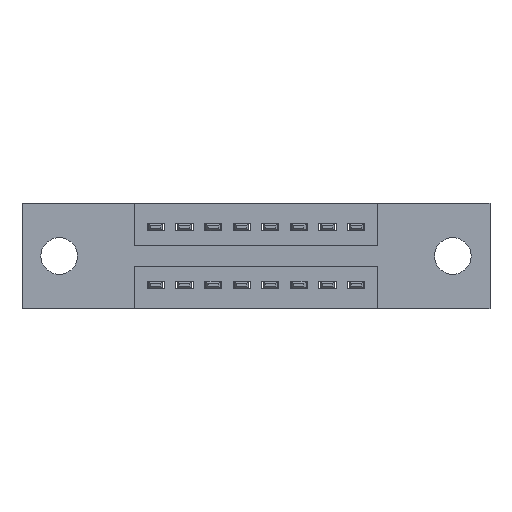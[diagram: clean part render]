
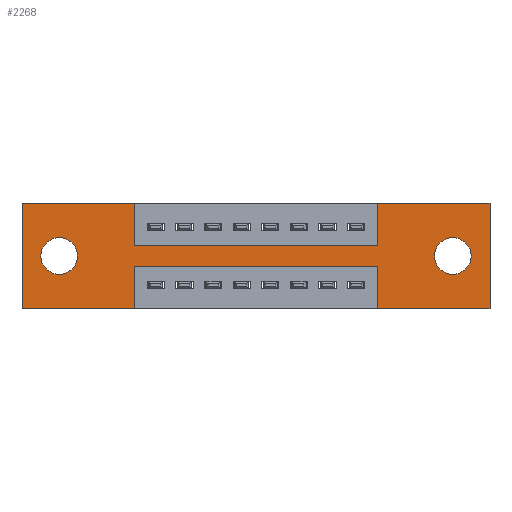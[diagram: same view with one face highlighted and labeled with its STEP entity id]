
A CAD part, front view. The second image highlights one B-rep face of the part: STEP entity #2268.
In plain terms, the highlighted planar face has unit normal (0, -1, 0).
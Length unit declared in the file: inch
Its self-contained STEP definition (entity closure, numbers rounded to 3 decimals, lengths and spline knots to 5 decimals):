
#105 = CARTESIAN_POINT ( 'NONE',  ( 0.3925, 0., -0.15 ) ) ;
#108 = CARTESIAN_POINT ( 'NONE',  ( 0.13, 0., -0.121 ) ) ;
#109 = FACE_BOUND ( 'NONE', #9488, .T. ) ;
#119 = DIRECTION ( 'NONE',  ( 0., -1., 0. ) ) ;
#205 = VERTEX_POINT ( 'NONE', #1158 ) ;
#261 = CARTESIAN_POINT ( 'NONE',  ( 0.13, 0., -0.249 ) ) ;
#336 = ORIENTED_EDGE ( 'NONE', *, *, #9798, .T. ) ;
#409 = CARTESIAN_POINT ( 'NONE',  ( 1.505, 0., -0.249 ) ) ;
#481 = DIRECTION ( 'NONE',  ( 1., 0., 0. ) ) ;
#488 = ORIENTED_EDGE ( 'NONE', *, *, #3546, .T. ) ;
#514 = LINE ( 'NONE', #9756, #5161 ) ;
#735 = CARTESIAN_POINT ( 'NONE',  ( 1.2425, 0., -0.37 ) ) ;
#747 = DIRECTION ( 'NONE',  ( 0., 0., -1. ) ) ;
#782 = DIRECTION ( 'NONE',  ( 0., 1., 0. ) ) ;
#883 = ORIENTED_EDGE ( 'NONE', *, *, #3444, .T. ) ;
#1049 = CARTESIAN_POINT ( 'NONE',  ( 0.3925, 0., 0. ) ) ;
#1069 = ORIENTED_EDGE ( 'NONE', *, *, #6286, .T. ) ;
#1088 = AXIS2_PLACEMENT_3D ( 'NONE', #8961, #8933, #3361 ) ;
#1124 = LINE ( 'NONE', #8609, #5435 ) ;
#1139 = EDGE_CURVE ( 'NONE', #6554, #6584, #8208, .T. ) ;
#1158 = CARTESIAN_POINT ( 'NONE',  ( 1.635, 0., -0.37 ) ) ;
#1349 = CARTESIAN_POINT ( 'NONE',  ( 1.505, 0., -0.185 ) ) ;
#1469 = EDGE_CURVE ( 'NONE', #1929, #6581, #5214, .T. ) ;
#1492 = VECTOR ( 'NONE', #3871, 39.37008 ) ;
#1554 = CARTESIAN_POINT ( 'NONE',  ( 1.2425, 0., -0.37 ) ) ;
#1603 = CIRCLE ( 'NONE', #6537, 0.064 ) ;
#1689 = CIRCLE ( 'NONE', #8355, 0.064 ) ;
#1772 = DIRECTION ( 'NONE',  ( 0., 0., 1. ) ) ;
#1795 = ORIENTED_EDGE ( 'NONE', *, *, #5296, .F. ) ;
#1887 = EDGE_CURVE ( 'NONE', #6584, #9141, #3772, .T. ) ;
#1929 = VERTEX_POINT ( 'NONE', #10676 ) ;
#1947 = VERTEX_POINT ( 'NONE', #261 ) ;
#2009 = EDGE_CURVE ( 'NONE', #8185, #10488, #4673, .T. ) ;
#2061 = ORIENTED_EDGE ( 'NONE', *, *, #1469, .F. ) ;
#2156 = ORIENTED_EDGE ( 'NONE', *, *, #2302, .F. ) ;
#2198 = ORIENTED_EDGE ( 'NONE', *, *, #3148, .F. ) ;
#2257 = DIRECTION ( 'NONE',  ( 0., 0., -1. ) ) ;
#2268 = ADVANCED_FACE ( 'NONE', ( #109, #2272, #6716 ), #5125, .T. ) ;
#2272 = FACE_BOUND ( 'NONE', #4322, .T. ) ;
#2302 = EDGE_CURVE ( 'NONE', #8116, #1929, #10304, .T. ) ;
#2501 = ORIENTED_EDGE ( 'NONE', *, *, #7516, .F. ) ;
#2599 = DIRECTION ( 'NONE',  ( 0., 0., -1. ) ) ;
#2653 = CARTESIAN_POINT ( 'NONE',  ( 1.2425, 0., 0. ) ) ;
#2776 = ORIENTED_EDGE ( 'NONE', *, *, #2009, .F. ) ;
#2954 = CARTESIAN_POINT ( 'NONE',  ( 0.3925, 0., 0. ) ) ;
#2968 = DIRECTION ( 'NONE',  ( 0., 0., 1. ) ) ;
#3147 = ORIENTED_EDGE ( 'NONE', *, *, #5895, .F. ) ;
#3148 = EDGE_CURVE ( 'NONE', #205, #8116, #6696, .T. ) ;
#3301 = ORIENTED_EDGE ( 'NONE', *, *, #1887, .F. ) ;
#3313 = ORIENTED_EDGE ( 'NONE', *, *, #1139, .F. ) ;
#3316 = CARTESIAN_POINT ( 'NONE',  ( 0.3925, 0., -0.37 ) ) ;
#3361 = DIRECTION ( 'NONE',  ( 0., 0., -1. ) ) ;
#3444 = EDGE_CURVE ( 'NONE', #8309, #1947, #8162, .T. ) ;
#3546 = EDGE_CURVE ( 'NONE', #7913, #3805, #6931, .T. ) ;
#3663 = VECTOR ( 'NONE', #747, 39.37008 ) ;
#3709 = ORIENTED_EDGE ( 'NONE', *, *, #8189, .F. ) ;
#3745 = VECTOR ( 'NONE', #1772, 39.37008 ) ;
#3772 = LINE ( 'NONE', #105, #5699 ) ;
#3793 = CARTESIAN_POINT ( 'NONE',  ( 0.3925, 0., -0.37 ) ) ;
#3805 = VERTEX_POINT ( 'NONE', #5075 ) ;
#3837 = CARTESIAN_POINT ( 'NONE',  ( 0.3925, 0., -0.15 ) ) ;
#3871 = DIRECTION ( 'NONE',  ( 0., 0., -1. ) ) ;
#3965 = VECTOR ( 'NONE', #4348, 39.37008 ) ;
#3995 = LINE ( 'NONE', #9830, #3745 ) ;
#4322 = EDGE_LOOP ( 'NONE', ( #883, #1069 ) ) ;
#4336 = ORIENTED_EDGE ( 'NONE', *, *, #6980, .F. ) ;
#4348 = DIRECTION ( 'NONE',  ( 1., 0., 0. ) ) ;
#4493 = VERTEX_POINT ( 'NONE', #8219 ) ;
#4520 = VECTOR ( 'NONE', #9313, 39.37008 ) ;
#4601 = VERTEX_POINT ( 'NONE', #7735 ) ;
#4673 = LINE ( 'NONE', #10606, #7091 ) ;
#4865 = LINE ( 'NONE', #8209, #7015 ) ;
#5075 = CARTESIAN_POINT ( 'NONE',  ( 1.505, 0., -0.121 ) ) ;
#5125 = PLANE ( 'NONE',  #9767 ) ;
#5161 = VECTOR ( 'NONE', #2599, 39.37008 ) ;
#5214 = LINE ( 'NONE', #9081, #5464 ) ;
#5296 = EDGE_CURVE ( 'NONE', #6581, #7438, #7876, .T. ) ;
#5390 = ORIENTED_EDGE ( 'NONE', *, *, #8733, .F. ) ;
#5435 = VECTOR ( 'NONE', #2968, 39.37008 ) ;
#5464 = VECTOR ( 'NONE', #9623, 39.37008 ) ;
#5699 = VECTOR ( 'NONE', #481, 39.37008 ) ;
#5827 = CARTESIAN_POINT ( 'NONE',  ( 1.635, 0., 0. ) ) ;
#5895 = EDGE_CURVE ( 'NONE', #9141, #8185, #1124, .T. ) ;
#5936 = CARTESIAN_POINT ( 'NONE',  ( 0.13, 0., -0.185 ) ) ;
#6159 = LINE ( 'NONE', #10601, #3965 ) ;
#6286 = EDGE_CURVE ( 'NONE', #1947, #8309, #1689, .T. ) ;
#6455 = VECTOR ( 'NONE', #6826, 39.37008 ) ;
#6537 = AXIS2_PLACEMENT_3D ( 'NONE', #1349, #7232, #2257 ) ;
#6554 = VERTEX_POINT ( 'NONE', #2954 ) ;
#6581 = VERTEX_POINT ( 'NONE', #8629 ) ;
#6584 = VERTEX_POINT ( 'NONE', #3837 ) ;
#6626 = DIRECTION ( 'NONE',  ( -1., 0., 0. ) ) ;
#6696 = LINE ( 'NONE', #9299, #4520 ) ;
#6716 = FACE_OUTER_BOUND ( 'NONE', #7766, .T. ) ;
#6740 = DIRECTION ( 'NONE',  ( 0., 0., 1. ) ) ;
#6784 = DIRECTION ( 'NONE',  ( 0., 0., -1. ) ) ;
#6826 = DIRECTION ( 'NONE',  ( 0., 0., 1. ) ) ;
#6931 = CIRCLE ( 'NONE', #1088, 0.064 ) ;
#6966 = AXIS2_PLACEMENT_3D ( 'NONE', #9503, #10080, #9565 ) ;
#6980 = EDGE_CURVE ( 'NONE', #4493, #4601, #3995, .T. ) ;
#7015 = VECTOR ( 'NONE', #6626, 39.37008 ) ;
#7091 = VECTOR ( 'NONE', #10526, 39.37008 ) ;
#7232 = DIRECTION ( 'NONE',  ( 0., 1., 0. ) ) ;
#7438 = VERTEX_POINT ( 'NONE', #3316 ) ;
#7516 = EDGE_CURVE ( 'NONE', #10488, #205, #514, .T. ) ;
#7735 = CARTESIAN_POINT ( 'NONE',  ( 0., 0., 0. ) ) ;
#7766 = EDGE_LOOP ( 'NONE', ( #1795, #2061, #2156, #2198, #2501, #2776, #3147, #3301, #3313, #3709, #4336, #5390 ) ) ;
#7876 = LINE ( 'NONE', #3793, #1492 ) ;
#7894 = CARTESIAN_POINT ( 'NONE',  ( 0., 0., -0.37 ) ) ;
#7913 = VERTEX_POINT ( 'NONE', #409 ) ;
#8116 = VERTEX_POINT ( 'NONE', #735 ) ;
#8162 = CIRCLE ( 'NONE', #6966, 0.064 ) ;
#8185 = VERTEX_POINT ( 'NONE', #2653 ) ;
#8189 = EDGE_CURVE ( 'NONE', #4601, #6554, #6159, .T. ) ;
#8208 = LINE ( 'NONE', #1049, #3663 ) ;
#8209 = CARTESIAN_POINT ( 'NONE',  ( 0., 0., -0.37 ) ) ;
#8219 = CARTESIAN_POINT ( 'NONE',  ( 0., 0., -0.37 ) ) ;
#8309 = VERTEX_POINT ( 'NONE', #108 ) ;
#8355 = AXIS2_PLACEMENT_3D ( 'NONE', #5936, #782, #6740 ) ;
#8609 = CARTESIAN_POINT ( 'NONE',  ( 1.2425, 0., 0. ) ) ;
#8629 = CARTESIAN_POINT ( 'NONE',  ( 0.3925, 0., -0.22 ) ) ;
#8716 = CARTESIAN_POINT ( 'NONE',  ( 1.2425, 0., -0.15 ) ) ;
#8733 = EDGE_CURVE ( 'NONE', #7438, #4493, #4865, .T. ) ;
#8933 = DIRECTION ( 'NONE',  ( 0., 1., 0. ) ) ;
#8961 = CARTESIAN_POINT ( 'NONE',  ( 1.505, 0., -0.185 ) ) ;
#9081 = CARTESIAN_POINT ( 'NONE',  ( 0.3925, 0., -0.22 ) ) ;
#9141 = VERTEX_POINT ( 'NONE', #8716 ) ;
#9299 = CARTESIAN_POINT ( 'NONE',  ( 0., 0., -0.37 ) ) ;
#9313 = DIRECTION ( 'NONE',  ( -1., 0., 0. ) ) ;
#9488 = EDGE_LOOP ( 'NONE', ( #336, #488 ) ) ;
#9503 = CARTESIAN_POINT ( 'NONE',  ( 0.13, 0., -0.185 ) ) ;
#9565 = DIRECTION ( 'NONE',  ( 0., 0., 1. ) ) ;
#9623 = DIRECTION ( 'NONE',  ( -1., 0., 0. ) ) ;
#9756 = CARTESIAN_POINT ( 'NONE',  ( 1.635, 0., 0. ) ) ;
#9767 = AXIS2_PLACEMENT_3D ( 'NONE', #7894, #119, #6784 ) ;
#9798 = EDGE_CURVE ( 'NONE', #3805, #7913, #1603, .T. ) ;
#9830 = CARTESIAN_POINT ( 'NONE',  ( 0., 0., 0. ) ) ;
#10080 = DIRECTION ( 'NONE',  ( 0., 1., 0. ) ) ;
#10304 = LINE ( 'NONE', #1554, #6455 ) ;
#10488 = VERTEX_POINT ( 'NONE', #5827 ) ;
#10526 = DIRECTION ( 'NONE',  ( 1., 0., 0. ) ) ;
#10601 = CARTESIAN_POINT ( 'NONE',  ( 0., 0., 0. ) ) ;
#10606 = CARTESIAN_POINT ( 'NONE',  ( 0., 0., 0. ) ) ;
#10676 = CARTESIAN_POINT ( 'NONE',  ( 1.2425, 0., -0.22 ) ) ;
